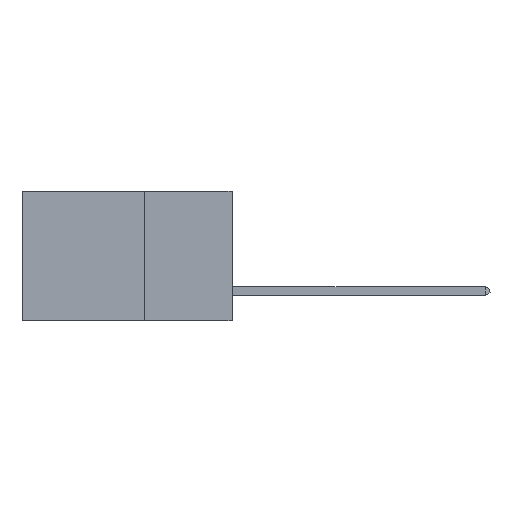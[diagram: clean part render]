
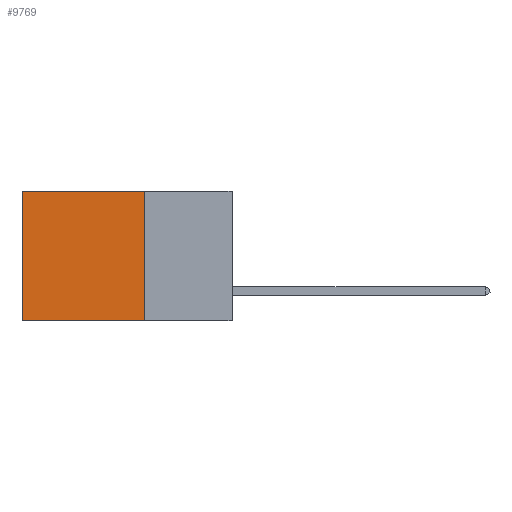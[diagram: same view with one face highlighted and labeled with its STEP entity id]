
A CAD part, left-side view. The second image highlights one B-rep face of the part: STEP entity #9769.
In plain terms, the highlighted planar face has unit normal (-1, 0, 0).
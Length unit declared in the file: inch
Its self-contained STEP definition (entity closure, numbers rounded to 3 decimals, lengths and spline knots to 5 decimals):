
#210 = EDGE_CURVE ( 'NONE', #32232, #9005, #22786, .T. ) ;
#261 = LINE ( 'NONE', #24840, #30199 ) ;
#1457 = VECTOR ( 'NONE', #8848, 39.37008 ) ;
#1480 = DIRECTION ( 'NONE',  ( 1., 0., 0. ) ) ;
#1755 = AXIS2_PLACEMENT_3D ( 'NONE', #7478, #1480, #12605 ) ;
#3260 = ORIENTED_EDGE ( 'NONE', *, *, #210, .T. ) ;
#4202 = EDGE_CURVE ( 'NONE', #32264, #9005, #14092, .T. ) ;
#6275 = EDGE_LOOP ( 'NONE', ( #3260, #13487, #9086, #30519 ) ) ;
#7478 = CARTESIAN_POINT ( 'NONE',  ( 0.2875, 0.25, 0. ) ) ;
#8848 = DIRECTION ( 'NONE',  ( 0., 1., 0. ) ) ;
#9005 = VERTEX_POINT ( 'NONE', #32148 ) ;
#9086 = ORIENTED_EDGE ( 'NONE', *, *, #21418, .F. ) ;
#9769 = ADVANCED_FACE ( 'NONE', ( #31542 ), #26072, .F. ) ;
#10988 = VERTEX_POINT ( 'NONE', #22621 ) ;
#12605 = DIRECTION ( 'NONE',  ( 0., 0., -1. ) ) ;
#13487 = ORIENTED_EDGE ( 'NONE', *, *, #4202, .F. ) ;
#13748 = CARTESIAN_POINT ( 'NONE',  ( 0.2875, 0.25, -0.37 ) ) ;
#14092 = LINE ( 'NONE', #13748, #21715 ) ;
#14347 = CARTESIAN_POINT ( 'NONE',  ( 0.2875, 0.25, 0. ) ) ;
#16940 = CARTESIAN_POINT ( 'NONE',  ( 0.2875, 0.6, 0. ) ) ;
#21418 = EDGE_CURVE ( 'NONE', #10988, #32264, #261, .T. ) ;
#21715 = VECTOR ( 'NONE', #21883, 39.37008 ) ;
#21883 = DIRECTION ( 'NONE',  ( 0., 1., 0. ) ) ;
#22308 = LINE ( 'NONE', #14347, #1457 ) ;
#22621 = CARTESIAN_POINT ( 'NONE',  ( 0.2875, 0.25, 0. ) ) ;
#22786 = LINE ( 'NONE', #16940, #24085 ) ;
#22892 = EDGE_CURVE ( 'NONE', #10988, #32232, #22308, .T. ) ;
#24085 = VECTOR ( 'NONE', #33573, 39.37008 ) ;
#24840 = CARTESIAN_POINT ( 'NONE',  ( 0.2875, 0.25, 0. ) ) ;
#25942 = CARTESIAN_POINT ( 'NONE',  ( 0.2875, 0.6, 0. ) ) ;
#26072 = PLANE ( 'NONE',  #1755 ) ;
#28606 = CARTESIAN_POINT ( 'NONE',  ( 0.2875, 0.25, -0.37 ) ) ;
#30199 = VECTOR ( 'NONE', #32974, 39.37008 ) ;
#30519 = ORIENTED_EDGE ( 'NONE', *, *, #22892, .T. ) ;
#31542 = FACE_OUTER_BOUND ( 'NONE', #6275, .T. ) ;
#32148 = CARTESIAN_POINT ( 'NONE',  ( 0.2875, 0.6, -0.37 ) ) ;
#32232 = VERTEX_POINT ( 'NONE', #25942 ) ;
#32264 = VERTEX_POINT ( 'NONE', #28606 ) ;
#32974 = DIRECTION ( 'NONE',  ( 0., 0., -1. ) ) ;
#33573 = DIRECTION ( 'NONE',  ( 0., 0., -1. ) ) ;
